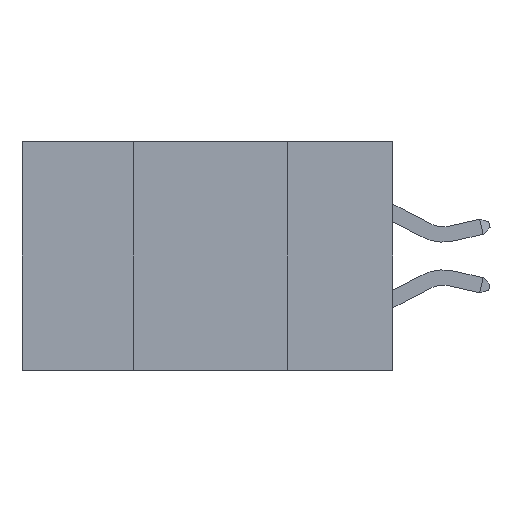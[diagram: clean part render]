
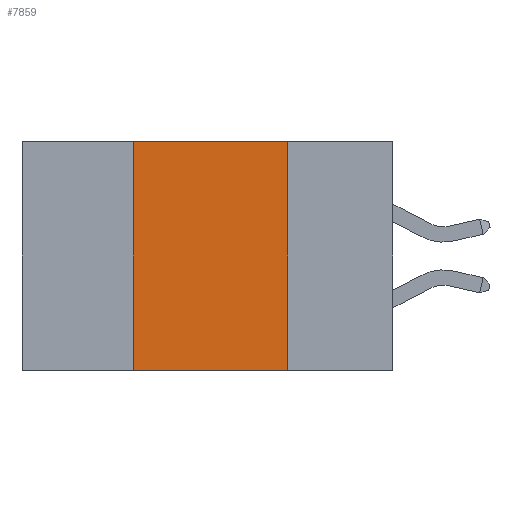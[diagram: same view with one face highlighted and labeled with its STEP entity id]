
A CAD part, left-side view. The second image highlights one B-rep face of the part: STEP entity #7859.
In plain terms, the highlighted planar face has unit normal (-1, 0, 0).
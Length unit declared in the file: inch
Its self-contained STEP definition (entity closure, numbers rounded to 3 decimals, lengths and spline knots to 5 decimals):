
#192 = CARTESIAN_POINT ( 'NONE',  ( 0., 0.42, 0. ) ) ;
#223 = CARTESIAN_POINT ( 'NONE',  ( 0., 0.42, -0.37 ) ) ;
#295 = ORIENTED_EDGE ( 'NONE', *, *, #17767, .T. ) ;
#779 = DIRECTION ( 'NONE',  ( 0., -1., 0. ) ) ;
#1713 = EDGE_CURVE ( 'NONE', #24891, #1726, #9820, .T. ) ;
#1726 = VERTEX_POINT ( 'NONE', #23502 ) ;
#3312 = DIRECTION ( 'NONE',  ( 0., -1., 0. ) ) ;
#4158 = DIRECTION ( 'NONE',  ( 0., 0., -1. ) ) ;
#4352 = CARTESIAN_POINT ( 'NONE',  ( 0., 0.17, 0. ) ) ;
#4400 = PLANE ( 'NONE',  #21127 ) ;
#5472 = EDGE_CURVE ( 'NONE', #21285, #6022, #21903, .T. ) ;
#6022 = VERTEX_POINT ( 'NONE', #10057 ) ;
#6341 = FACE_OUTER_BOUND ( 'NONE', #19958, .T. ) ;
#7859 = ADVANCED_FACE ( 'NONE', ( #6341 ), #4400, .F. ) ;
#8267 = DIRECTION ( 'NONE',  ( 1., 0., 0. ) ) ;
#9820 = LINE ( 'NONE', #192, #13864 ) ;
#10057 = CARTESIAN_POINT ( 'NONE',  ( 0., 0.17, -0.37 ) ) ;
#10662 = CARTESIAN_POINT ( 'NONE',  ( 0., 0.6, 0. ) ) ;
#11294 = VECTOR ( 'NONE', #779, 39.37008 ) ;
#11835 = CARTESIAN_POINT ( 'NONE',  ( 0., 0.17, 0. ) ) ;
#12197 = DIRECTION ( 'NONE',  ( 0., 0., -1. ) ) ;
#13074 = LINE ( 'NONE', #24835, #21420 ) ;
#13494 = ORIENTED_EDGE ( 'NONE', *, *, #20211, .F. ) ;
#13547 = DIRECTION ( 'NONE',  ( 0., 0., 1. ) ) ;
#13864 = VECTOR ( 'NONE', #13547, 39.37008 ) ;
#17767 = EDGE_CURVE ( 'NONE', #24891, #6022, #13074, .T. ) ;
#19958 = EDGE_LOOP ( 'NONE', ( #24282, #13494, #25227, #295 ) ) ;
#20047 = CARTESIAN_POINT ( 'NONE',  ( 0., 0.6, 0. ) ) ;
#20211 = EDGE_CURVE ( 'NONE', #1726, #21285, #20372, .T. ) ;
#20372 = LINE ( 'NONE', #10662, #11294 ) ;
#20874 = VECTOR ( 'NONE', #12197, 39.37008 ) ;
#21127 = AXIS2_PLACEMENT_3D ( 'NONE', #20047, #8267, #4158 ) ;
#21285 = VERTEX_POINT ( 'NONE', #11835 ) ;
#21420 = VECTOR ( 'NONE', #3312, 39.37008 ) ;
#21903 = LINE ( 'NONE', #4352, #20874 ) ;
#23502 = CARTESIAN_POINT ( 'NONE',  ( 0., 0.42, 0. ) ) ;
#24282 = ORIENTED_EDGE ( 'NONE', *, *, #5472, .F. ) ;
#24835 = CARTESIAN_POINT ( 'NONE',  ( 0., 0.6, -0.37 ) ) ;
#24891 = VERTEX_POINT ( 'NONE', #223 ) ;
#25227 = ORIENTED_EDGE ( 'NONE', *, *, #1713, .F. ) ;
